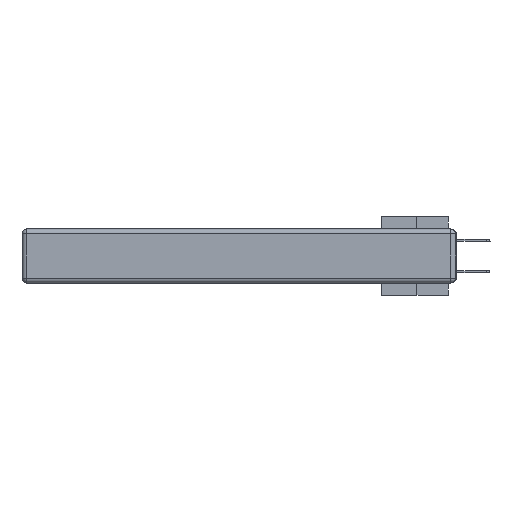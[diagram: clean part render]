
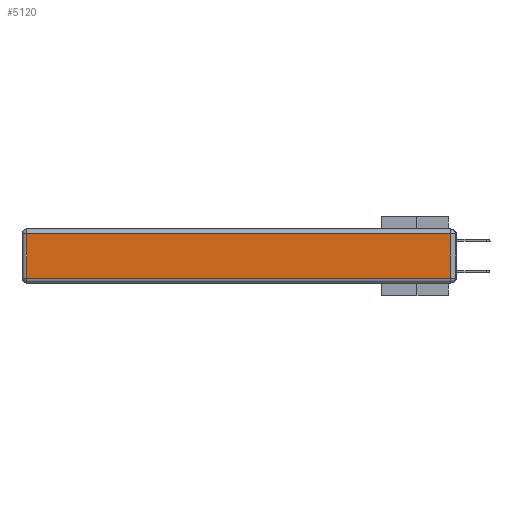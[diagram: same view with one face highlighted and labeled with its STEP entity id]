
A CAD part, left-side view. The second image highlights one B-rep face of the part: STEP entity #5120.
In plain terms, the highlighted planar face has unit normal (-1, 0, 0).
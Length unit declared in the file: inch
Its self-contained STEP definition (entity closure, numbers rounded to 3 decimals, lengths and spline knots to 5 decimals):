
#412 = CARTESIAN_POINT ( 'NONE',  ( 0., 0.03, -0.313 ) ) ;
#1446 = VERTEX_POINT ( 'NONE', #11940 ) ;
#1760 = EDGE_CURVE ( 'NONE', #17127, #10594, #18747, .T. ) ;
#3003 = EDGE_CURVE ( 'NONE', #10594, #1446, #27320, .T. ) ;
#3753 = DIRECTION ( 'NONE',  ( 0., 0., 1. ) ) ;
#4291 = FACE_OUTER_BOUND ( 'NONE', #19036, .T. ) ;
#4704 = VECTOR ( 'NONE', #19945, 39.37008 ) ;
#4944 = EDGE_CURVE ( 'NONE', #25818, #17127, #24777, .T. ) ;
#5120 = ADVANCED_FACE ( 'NONE', ( #4291 ), #6812, .T. ) ;
#5323 = ORIENTED_EDGE ( 'NONE', *, *, #3003, .T. ) ;
#6804 = DIRECTION ( 'NONE',  ( 0., 0., 1. ) ) ;
#6812 = PLANE ( 'NONE',  #16208 ) ;
#10177 = VECTOR ( 'NONE', #6804, 39.37008 ) ;
#10594 = VERTEX_POINT ( 'NONE', #12170 ) ;
#11650 = VECTOR ( 'NONE', #13714, 39.37008 ) ;
#11940 = CARTESIAN_POINT ( 'NONE',  ( 0., 2.72, -0.03 ) ) ;
#12170 = CARTESIAN_POINT ( 'NONE',  ( 0., 0.03, -0.03 ) ) ;
#12947 = CARTESIAN_POINT ( 'NONE',  ( 0., 2.72, -0.343 ) ) ;
#13299 = LINE ( 'NONE', #12947, #29926 ) ;
#13714 = DIRECTION ( 'NONE',  ( 0., 1., 0. ) ) ;
#15099 = ORIENTED_EDGE ( 'NONE', *, *, #1760, .T. ) ;
#16208 = AXIS2_PLACEMENT_3D ( 'NONE', #31074, #23158, #3753 ) ;
#17127 = VERTEX_POINT ( 'NONE', #412 ) ;
#18747 = LINE ( 'NONE', #29689, #10177 ) ;
#19036 = EDGE_LOOP ( 'NONE', ( #23490, #15099, #5323, #20134 ) ) ;
#19945 = DIRECTION ( 'NONE',  ( 0., -1., 0. ) ) ;
#20134 = ORIENTED_EDGE ( 'NONE', *, *, #22331, .T. ) ;
#22331 = EDGE_CURVE ( 'NONE', #1446, #25818, #13299, .T. ) ;
#22810 = CARTESIAN_POINT ( 'NONE',  ( 0., 0., -0.313 ) ) ;
#23158 = DIRECTION ( 'NONE',  ( -1., 0., 0. ) ) ;
#23490 = ORIENTED_EDGE ( 'NONE', *, *, #4944, .T. ) ;
#24777 = LINE ( 'NONE', #22810, #4704 ) ;
#25818 = VERTEX_POINT ( 'NONE', #33041 ) ;
#26728 = DIRECTION ( 'NONE',  ( 0., 0., -1. ) ) ;
#27144 = CARTESIAN_POINT ( 'NONE',  ( 0., 2.75, -0.03 ) ) ;
#27320 = LINE ( 'NONE', #27144, #11650 ) ;
#29689 = CARTESIAN_POINT ( 'NONE',  ( 0., 0.03, -0.343 ) ) ;
#29926 = VECTOR ( 'NONE', #26728, 39.37008 ) ;
#31074 = CARTESIAN_POINT ( 'NONE',  ( 0., 0., -0.343 ) ) ;
#33041 = CARTESIAN_POINT ( 'NONE',  ( 0., 2.72, -0.313 ) ) ;
